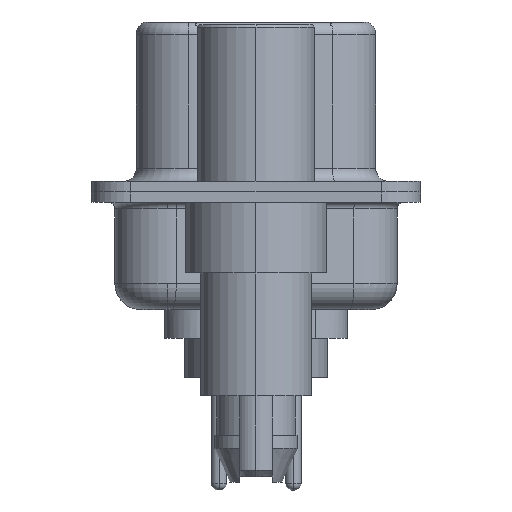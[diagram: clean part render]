
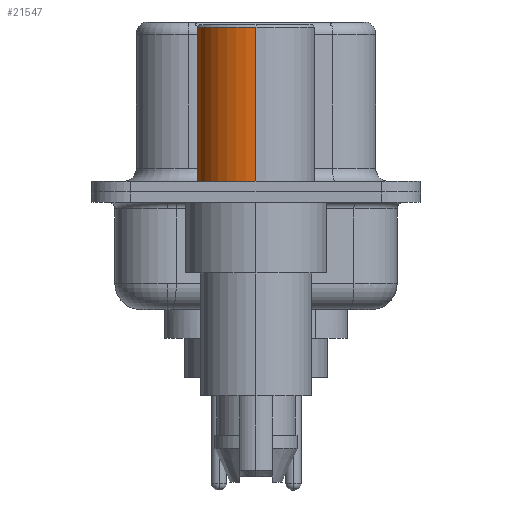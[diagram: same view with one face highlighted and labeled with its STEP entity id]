
A CAD part, left-side view. The second image highlights one B-rep face of the part: STEP entity #21547.
In plain terms, the highlighted cylindrical face has radius 2.25 mm (diameter 4.5 mm), a partial arc.
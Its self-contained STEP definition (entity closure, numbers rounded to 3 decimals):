
#544 = DIRECTION ( 'NONE',  ( 1., 0., 0. ) ) ;
#1021 = ORIENTED_EDGE ( 'NONE', *, *, #8912, .T. ) ;
#2557 = CARTESIAN_POINT ( 'NONE',  ( 0., 0., 0.4 ) ) ;
#2594 = VECTOR ( 'NONE', #3089, 1000. ) ;
#3089 = DIRECTION ( 'NONE',  ( 0., 0., 1. ) ) ;
#3814 = VECTOR ( 'NONE', #11762, 1000. ) ;
#3867 = CARTESIAN_POINT ( 'NONE',  ( 0., 0., 0.581 ) ) ;
#4262 = DIRECTION ( 'NONE',  ( 1., 0., 0. ) ) ;
#5247 = FACE_OUTER_BOUND ( 'NONE', #10474, .T. ) ;
#5586 = AXIS2_PLACEMENT_3D ( 'NONE', #2557, #14275, #4262 ) ;
#7132 = VERTEX_POINT ( 'NONE', #7562 ) ;
#7345 = CARTESIAN_POINT ( 'NONE',  ( -2.25, 0., 6.3 ) ) ;
#7562 = CARTESIAN_POINT ( 'NONE',  ( 2.25, 0., 0.4 ) ) ;
#8912 = EDGE_CURVE ( 'NONE', #10299, #19810, #16013, .T. ) ;
#9451 = ORIENTED_EDGE ( 'NONE', *, *, #15121, .F. ) ;
#10299 = VERTEX_POINT ( 'NONE', #10341 ) ;
#10341 = CARTESIAN_POINT ( 'NONE',  ( -2.25, 0., 0.4 ) ) ;
#10474 = EDGE_LOOP ( 'NONE', ( #16871, #1021, #9451, #20700 ) ) ;
#10566 = DIRECTION ( 'NONE',  ( 0., 0., 1. ) ) ;
#11762 = DIRECTION ( 'NONE',  ( 0., 0., 1. ) ) ;
#11838 = CIRCLE ( 'NONE', #14586, 2.25 ) ;
#12173 = DIRECTION ( 'NONE',  ( 1., 0., 0. ) ) ;
#13763 = LINE ( 'NONE', #15281, #3814 ) ;
#13985 = EDGE_CURVE ( 'NONE', #7132, #10299, #17946, .T. ) ;
#14275 = DIRECTION ( 'NONE',  ( 0., 0., 1. ) ) ;
#14586 = AXIS2_PLACEMENT_3D ( 'NONE', #20713, #10566, #544 ) ;
#15121 = EDGE_CURVE ( 'NONE', #20952, #19810, #11838, .T. ) ;
#15281 = CARTESIAN_POINT ( 'NONE',  ( 2.25, 0., 0.581 ) ) ;
#16013 = LINE ( 'NONE', #21683, #2594 ) ;
#16871 = ORIENTED_EDGE ( 'NONE', *, *, #13985, .T. ) ;
#16876 = AXIS2_PLACEMENT_3D ( 'NONE', #3867, #20731, #12173 ) ;
#17946 = CIRCLE ( 'NONE', #5586, 2.25 ) ;
#18134 = CYLINDRICAL_SURFACE ( 'NONE', #16876, 2.25 ) ;
#19269 = CARTESIAN_POINT ( 'NONE',  ( 2.25, 0., 6.3 ) ) ;
#19810 = VERTEX_POINT ( 'NONE', #7345 ) ;
#20700 = ORIENTED_EDGE ( 'NONE', *, *, #20833, .F. ) ;
#20713 = CARTESIAN_POINT ( 'NONE',  ( 0., 0., 6.3 ) ) ;
#20731 = DIRECTION ( 'NONE',  ( 0., 0., 1. ) ) ;
#20833 = EDGE_CURVE ( 'NONE', #7132, #20952, #13763, .T. ) ;
#20952 = VERTEX_POINT ( 'NONE', #19269 ) ;
#21547 = ADVANCED_FACE ( 'NONE', ( #5247 ), #18134, .T. ) ;
#21683 = CARTESIAN_POINT ( 'NONE',  ( -2.25, 0., 0.581 ) ) ;
